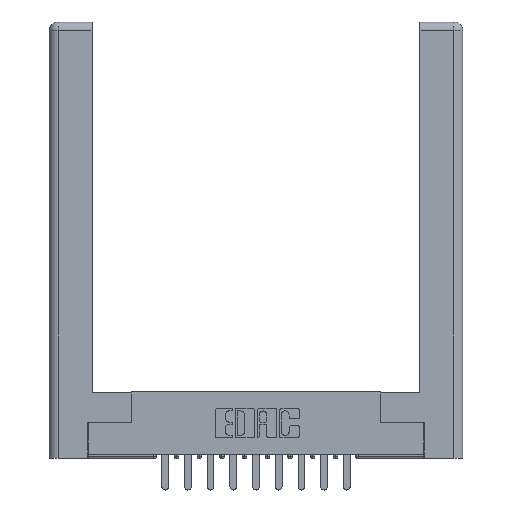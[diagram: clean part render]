
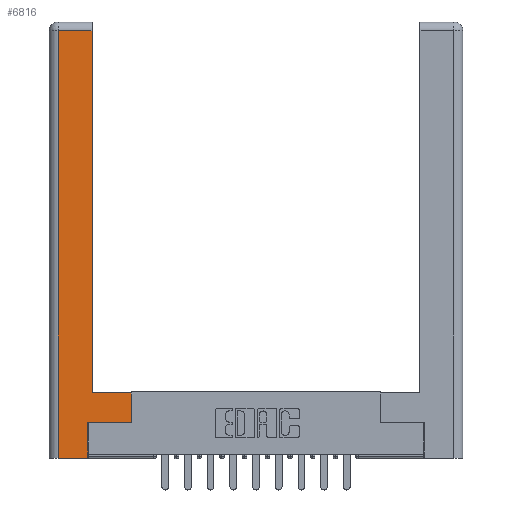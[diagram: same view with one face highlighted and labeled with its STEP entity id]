
A CAD part, top view. The second image highlights one B-rep face of the part: STEP entity #6816.
In plain terms, the highlighted planar face has unit normal (0, 0, 1).
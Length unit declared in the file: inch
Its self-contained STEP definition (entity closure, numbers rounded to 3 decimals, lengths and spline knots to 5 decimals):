
#607 = VECTOR ( 'NONE', #8299, 39.37008 ) ;
#1308 = DIRECTION ( 'NONE',  ( 0., 1., 0. ) ) ;
#1377 = CARTESIAN_POINT ( 'NONE',  ( 0.265, 0., 0. ) ) ;
#1441 = EDGE_CURVE ( 'NONE', #10668, #8120, #12782, .T. ) ;
#1458 = EDGE_CURVE ( 'NONE', #3903, #4841, #6325, .T. ) ;
#1527 = ORIENTED_EDGE ( 'NONE', *, *, #14902, .T. ) ;
#2098 = DIRECTION ( 'NONE',  ( 0., 0., -1. ) ) ;
#2564 = VECTOR ( 'NONE', #12535, 39.37008 ) ;
#2646 = CARTESIAN_POINT ( 'NONE',  ( 0.565, 0.45, 0. ) ) ;
#3428 = CARTESIAN_POINT ( 'NONE',  ( 0.265, 0.245, 0. ) ) ;
#3607 = CARTESIAN_POINT ( 'NONE',  ( 0.0615, 0., 0. ) ) ;
#3903 = VERTEX_POINT ( 'NONE', #10147 ) ;
#4377 = LINE ( 'NONE', #8351, #607 ) ;
#4450 = CARTESIAN_POINT ( 'NONE',  ( 0.565, 0.245, 0. ) ) ;
#4587 = ORIENTED_EDGE ( 'NONE', *, *, #11637, .T. ) ;
#4684 = LINE ( 'NONE', #10195, #10587 ) ;
#4841 = VERTEX_POINT ( 'NONE', #14459 ) ;
#4949 = VERTEX_POINT ( 'NONE', #5627 ) ;
#5059 = VECTOR ( 'NONE', #11433, 39.37008 ) ;
#5136 = ORIENTED_EDGE ( 'NONE', *, *, #1458, .T. ) ;
#5233 = CARTESIAN_POINT ( 'NONE',  ( 0.265, 0., 0. ) ) ;
#5627 = CARTESIAN_POINT ( 'NONE',  ( 0.295, 0.45, 0. ) ) ;
#5641 = CARTESIAN_POINT ( 'NONE',  ( 0.295, 3., 0. ) ) ;
#5754 = VERTEX_POINT ( 'NONE', #3607 ) ;
#6179 = VERTEX_POINT ( 'NONE', #4450 ) ;
#6281 = FACE_OUTER_BOUND ( 'NONE', #11678, .T. ) ;
#6325 = LINE ( 'NONE', #9506, #9468 ) ;
#6535 = VECTOR ( 'NONE', #6973, 39.37008 ) ;
#6816 = ADVANCED_FACE ( 'NONE', ( #6281 ), #13857, .F. ) ;
#6973 = DIRECTION ( 'NONE',  ( 0., -1., 0. ) ) ;
#7066 = CARTESIAN_POINT ( 'NONE',  ( 0., 0., 0. ) ) ;
#7314 = ORIENTED_EDGE ( 'NONE', *, *, #1441, .T. ) ;
#7856 = LINE ( 'NONE', #12546, #5059 ) ;
#8120 = VERTEX_POINT ( 'NONE', #3428 ) ;
#8270 = DIRECTION ( 'NONE',  ( -1., 0., 0. ) ) ;
#8299 = DIRECTION ( 'NONE',  ( 0., 1., 0. ) ) ;
#8351 = CARTESIAN_POINT ( 'NONE',  ( 0.565, 0.45, 0. ) ) ;
#8417 = VERTEX_POINT ( 'NONE', #2646 ) ;
#8467 = ORIENTED_EDGE ( 'NONE', *, *, #10851, .T. ) ;
#9302 = CARTESIAN_POINT ( 'NONE',  ( 0.0615, 0., 0. ) ) ;
#9468 = VECTOR ( 'NONE', #9912, 39.37008 ) ;
#9506 = CARTESIAN_POINT ( 'NONE',  ( 0.0615, 2.94, 0. ) ) ;
#9595 = ORIENTED_EDGE ( 'NONE', *, *, #14688, .T. ) ;
#9677 = LINE ( 'NONE', #9302, #6535 ) ;
#9791 = LINE ( 'NONE', #5233, #12032 ) ;
#9912 = DIRECTION ( 'NONE',  ( -1., 0., 0. ) ) ;
#10147 = CARTESIAN_POINT ( 'NONE',  ( 0.295, 2.94, 0. ) ) ;
#10195 = CARTESIAN_POINT ( 'NONE',  ( 0.295, 0.45, 0. ) ) ;
#10393 = ORIENTED_EDGE ( 'NONE', *, *, #13903, .T. ) ;
#10587 = VECTOR ( 'NONE', #11305, 39.37008 ) ;
#10668 = VERTEX_POINT ( 'NONE', #1377 ) ;
#10851 = EDGE_CURVE ( 'NONE', #8417, #4949, #4684, .T. ) ;
#10941 = CARTESIAN_POINT ( 'NONE',  ( 0.265, 0.245, 0. ) ) ;
#11046 = DIRECTION ( 'NONE',  ( 1., 0., 0. ) ) ;
#11305 = DIRECTION ( 'NONE',  ( -1., 0., 0. ) ) ;
#11433 = DIRECTION ( 'NONE',  ( 1., 0., 0. ) ) ;
#11637 = EDGE_CURVE ( 'NONE', #8120, #6179, #7856, .T. ) ;
#11678 = EDGE_LOOP ( 'NONE', ( #10393, #5136, #14408, #1527, #7314, #4587, #9595, #8467 ) ) ;
#12032 = VECTOR ( 'NONE', #11046, 39.37008 ) ;
#12330 = EDGE_CURVE ( 'NONE', #4841, #5754, #9677, .T. ) ;
#12427 = VECTOR ( 'NONE', #1308, 39.37008 ) ;
#12535 = DIRECTION ( 'NONE',  ( 0., 1., 0. ) ) ;
#12546 = CARTESIAN_POINT ( 'NONE',  ( 0.565, 0.245, 0. ) ) ;
#12782 = LINE ( 'NONE', #10941, #12427 ) ;
#12940 = AXIS2_PLACEMENT_3D ( 'NONE', #7066, #2098, #8270 ) ;
#13857 = PLANE ( 'NONE',  #12940 ) ;
#13903 = EDGE_CURVE ( 'NONE', #4949, #3903, #14952, .T. ) ;
#14408 = ORIENTED_EDGE ( 'NONE', *, *, #12330, .T. ) ;
#14459 = CARTESIAN_POINT ( 'NONE',  ( 0.0615, 2.94, 0. ) ) ;
#14688 = EDGE_CURVE ( 'NONE', #6179, #8417, #4377, .T. ) ;
#14902 = EDGE_CURVE ( 'NONE', #5754, #10668, #9791, .T. ) ;
#14952 = LINE ( 'NONE', #5641, #2564 ) ;
